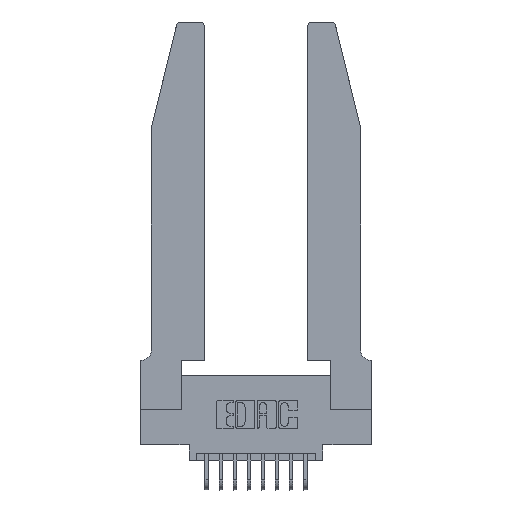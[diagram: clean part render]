
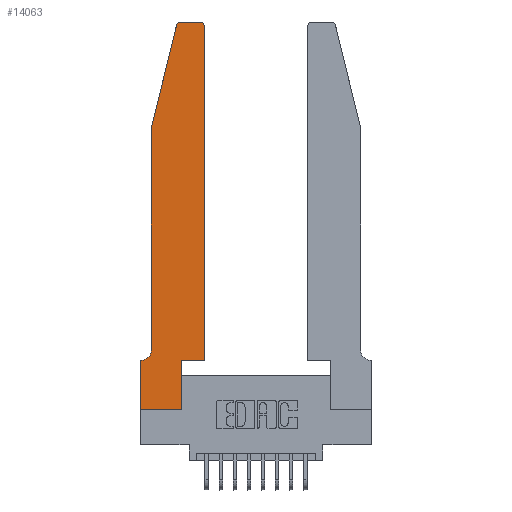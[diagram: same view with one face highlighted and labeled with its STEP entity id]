
A CAD part, top view. The second image highlights one B-rep face of the part: STEP entity #14063.
In plain terms, the highlighted planar face has unit normal (0, 0, 1).
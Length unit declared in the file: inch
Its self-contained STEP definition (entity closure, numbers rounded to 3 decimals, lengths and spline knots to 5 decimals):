
#471 = CARTESIAN_POINT ( 'NONE',  ( 0., 0.35, 0.37 ) ) ;
#518 = CARTESIAN_POINT ( 'NONE',  ( 0.4205, 2.75, 0.37 ) ) ;
#551 = EDGE_CURVE ( 'NONE', #13455, #9967, #9376, .T. ) ;
#1402 = ORIENTED_EDGE ( 'NONE', *, *, #2495, .T. ) ;
#1559 = DIRECTION ( 'NONE',  ( 0., -1., 0. ) ) ;
#1650 = LINE ( 'NONE', #12908, #12796 ) ;
#2028 = DIRECTION ( 'NONE',  ( 0., -1., 0. ) ) ;
#2160 = DIRECTION ( 'NONE',  ( 1., 0., 0. ) ) ;
#2238 = AXIS2_PLACEMENT_3D ( 'NONE', #471, #9892, #16580 ) ;
#2439 = ORIENTED_EDGE ( 'NONE', *, *, #9239, .T. ) ;
#2495 = EDGE_CURVE ( 'NONE', #16372, #14805, #12259, .T. ) ;
#2703 = CARTESIAN_POINT ( 'NONE',  ( 0.0755, 2., 0.37 ) ) ;
#2811 = ORIENTED_EDGE ( 'NONE', *, *, #10681, .T. ) ;
#2825 = EDGE_CURVE ( 'NONE', #16158, #6340, #14125, .T. ) ;
#3086 = ORIENTED_EDGE ( 'NONE', *, *, #4245, .T. ) ;
#3104 = VECTOR ( 'NONE', #2028, 39.37008 ) ;
#3202 = LINE ( 'NONE', #11859, #14963 ) ;
#3359 = CARTESIAN_POINT ( 'NONE',  ( 0.0755, 0.42, 0.37 ) ) ;
#3565 = DIRECTION ( 'NONE',  ( -1., 0., 0. ) ) ;
#3620 = EDGE_CURVE ( 'NONE', #9967, #5172, #3202, .T. ) ;
#3632 = EDGE_CURVE ( 'NONE', #14805, #14356, #14542, .T. ) ;
#3720 = CARTESIAN_POINT ( 'NONE',  ( 0.0755, 2., 0.37 ) ) ;
#3731 = CARTESIAN_POINT ( 'NONE',  ( 0.4505, 2.72, 0.37 ) ) ;
#4245 = EDGE_CURVE ( 'NONE', #6340, #11517, #14307, .T. ) ;
#4698 = CARTESIAN_POINT ( 'NONE',  ( 0.2865, 0., 0.37 ) ) ;
#5172 = VERTEX_POINT ( 'NONE', #4698 ) ;
#5191 = CARTESIAN_POINT ( 'NONE',  ( 0.4505, 0.35, 0.37 ) ) ;
#5368 = CARTESIAN_POINT ( 'NONE',  ( 0.2865, 0.35, 0.37 ) ) ;
#5662 = CARTESIAN_POINT ( 'NONE',  ( 0.0055, 0.35, 0.37 ) ) ;
#5727 = CARTESIAN_POINT ( 'NONE',  ( 0., 0.35, 0.37 ) ) ;
#6251 = FACE_OUTER_BOUND ( 'NONE', #7949, .T. ) ;
#6340 = VERTEX_POINT ( 'NONE', #12569 ) ;
#6467 = DIRECTION ( 'NONE',  ( 1., 0., 0. ) ) ;
#6531 = DIRECTION ( 'NONE',  ( 0., 1., 0. ) ) ;
#6593 = CIRCLE ( 'NONE', #7889, 0.03 ) ;
#6682 = ORIENTED_EDGE ( 'NONE', *, *, #13042, .T. ) ;
#7002 = VECTOR ( 'NONE', #10729, 39.37008 ) ;
#7388 = VECTOR ( 'NONE', #1559, 39.37008 ) ;
#7409 = CARTESIAN_POINT ( 'NONE',  ( 0.4205, 2.72, 0.37 ) ) ;
#7889 = AXIS2_PLACEMENT_3D ( 'NONE', #7409, #15401, #14155 ) ;
#7949 = EDGE_LOOP ( 'NONE', ( #15135, #2439, #14635, #3086, #9047, #6682, #16062, #16482, #2811, #1402, #12753, #13087 ) ) ;
#8100 = AXIS2_PLACEMENT_3D ( 'NONE', #9346, #13419, #16131 ) ;
#8289 = DIRECTION ( 'NONE',  ( 0., 1., 0. ) ) ;
#8597 = CARTESIAN_POINT ( 'NONE',  ( 0., 0., 0.37 ) ) ;
#8911 = CARTESIAN_POINT ( 'NONE',  ( 0.284, 2.72, 0.37 ) ) ;
#9047 = ORIENTED_EDGE ( 'NONE', *, *, #14807, .T. ) ;
#9229 = LINE ( 'NONE', #12875, #15132 ) ;
#9239 = EDGE_CURVE ( 'NONE', #10660, #16158, #15021, .T. ) ;
#9346 = CARTESIAN_POINT ( 'NONE',  ( 0.0055, 0.42, 0.37 ) ) ;
#9376 = LINE ( 'NONE', #8597, #3104 ) ;
#9892 = DIRECTION ( 'NONE',  ( 0., 0., 1. ) ) ;
#9967 = VERTEX_POINT ( 'NONE', #14689 ) ;
#10353 = DIRECTION ( 'NONE',  ( -1., 0., 0. ) ) ;
#10544 = DIRECTION ( 'NONE',  ( -0.239, -0.971, 0. ) ) ;
#10660 = VERTEX_POINT ( 'NONE', #17072 ) ;
#10681 = EDGE_CURVE ( 'NONE', #5172, #16372, #16020, .T. ) ;
#10729 = DIRECTION ( 'NONE',  ( 1., 0., 0. ) ) ;
#11277 = AXIS2_PLACEMENT_3D ( 'NONE', #8911, #16867, #2160 ) ;
#11480 = VERTEX_POINT ( 'NONE', #518 ) ;
#11517 = VERTEX_POINT ( 'NONE', #3359 ) ;
#11859 = CARTESIAN_POINT ( 'NONE',  ( 0., 0., 0.37 ) ) ;
#11995 = CARTESIAN_POINT ( 'NONE',  ( 0.4505, 0.35, 0.37 ) ) ;
#12073 = CARTESIAN_POINT ( 'NONE',  ( 0.2865, 0.35, 0.37 ) ) ;
#12259 = LINE ( 'NONE', #14264, #7002 ) ;
#12400 = EDGE_CURVE ( 'NONE', #11480, #10660, #9229, .T. ) ;
#12569 = CARTESIAN_POINT ( 'NONE',  ( 0.0755, 2., 0.37 ) ) ;
#12753 = ORIENTED_EDGE ( 'NONE', *, *, #3632, .T. ) ;
#12796 = VECTOR ( 'NONE', #10353, 39.37008 ) ;
#12875 = CARTESIAN_POINT ( 'NONE',  ( 0.2605, 2.75, 0.37 ) ) ;
#12908 = CARTESIAN_POINT ( 'NONE',  ( 0.0755, 0.35, 0.37 ) ) ;
#13042 = EDGE_CURVE ( 'NONE', #14975, #13455, #1650, .T. ) ;
#13075 = CARTESIAN_POINT ( 'NONE',  ( 0.25487, 2.72718, 0.37 ) ) ;
#13087 = ORIENTED_EDGE ( 'NONE', *, *, #17266, .T. ) ;
#13270 = VECTOR ( 'NONE', #8289, 39.37008 ) ;
#13419 = DIRECTION ( 'NONE',  ( 0., 0., -1. ) ) ;
#13455 = VERTEX_POINT ( 'NONE', #5727 ) ;
#14063 = ADVANCED_FACE ( 'NONE', ( #6251 ), #16754, .T. ) ;
#14125 = LINE ( 'NONE', #3720, #16882 ) ;
#14155 = DIRECTION ( 'NONE',  ( 1., 0., 0. ) ) ;
#14264 = CARTESIAN_POINT ( 'NONE',  ( 0.4505, 0.35, 0.37 ) ) ;
#14307 = LINE ( 'NONE', #2703, #7388 ) ;
#14356 = VERTEX_POINT ( 'NONE', #3731 ) ;
#14542 = LINE ( 'NONE', #5191, #15378 ) ;
#14635 = ORIENTED_EDGE ( 'NONE', *, *, #2825, .T. ) ;
#14689 = CARTESIAN_POINT ( 'NONE',  ( 0., 0., 0.37 ) ) ;
#14805 = VERTEX_POINT ( 'NONE', #11995 ) ;
#14807 = EDGE_CURVE ( 'NONE', #11517, #14975, #17186, .T. ) ;
#14963 = VECTOR ( 'NONE', #6467, 39.37008 ) ;
#14975 = VERTEX_POINT ( 'NONE', #5662 ) ;
#15021 = CIRCLE ( 'NONE', #11277, 0.03 ) ;
#15132 = VECTOR ( 'NONE', #3565, 39.37008 ) ;
#15135 = ORIENTED_EDGE ( 'NONE', *, *, #12400, .T. ) ;
#15378 = VECTOR ( 'NONE', #6531, 39.37008 ) ;
#15401 = DIRECTION ( 'NONE',  ( 0., 0., 1. ) ) ;
#16020 = LINE ( 'NONE', #5368, #13270 ) ;
#16062 = ORIENTED_EDGE ( 'NONE', *, *, #551, .T. ) ;
#16131 = DIRECTION ( 'NONE',  ( -1., 0., 0. ) ) ;
#16158 = VERTEX_POINT ( 'NONE', #13075 ) ;
#16372 = VERTEX_POINT ( 'NONE', #12073 ) ;
#16482 = ORIENTED_EDGE ( 'NONE', *, *, #3620, .T. ) ;
#16580 = DIRECTION ( 'NONE',  ( 1., 0., 0. ) ) ;
#16754 = PLANE ( 'NONE',  #2238 ) ;
#16867 = DIRECTION ( 'NONE',  ( 0., 0., 1. ) ) ;
#16882 = VECTOR ( 'NONE', #10544, 39.37008 ) ;
#17072 = CARTESIAN_POINT ( 'NONE',  ( 0.284, 2.75, 0.37 ) ) ;
#17186 = CIRCLE ( 'NONE', #8100, 0.07 ) ;
#17266 = EDGE_CURVE ( 'NONE', #14356, #11480, #6593, .T. ) ;
